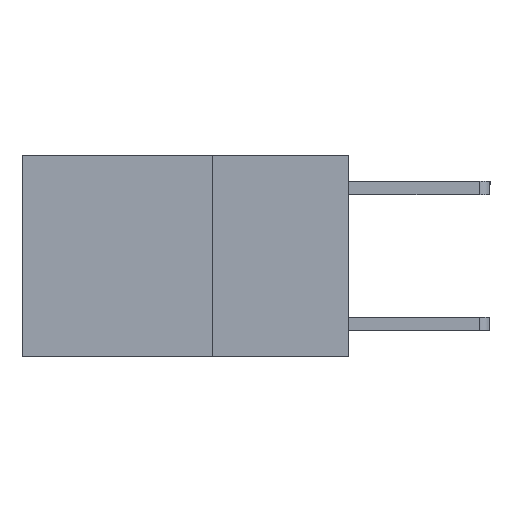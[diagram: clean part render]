
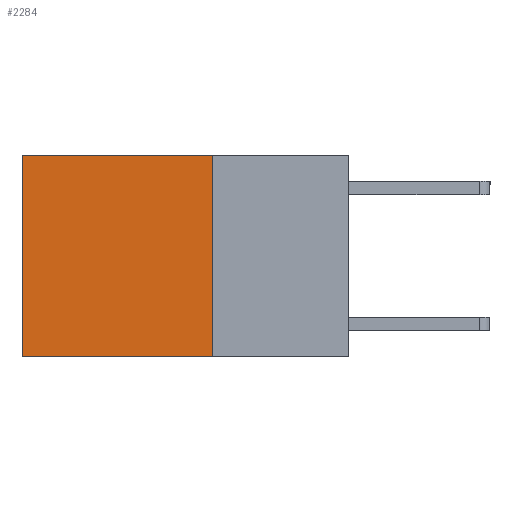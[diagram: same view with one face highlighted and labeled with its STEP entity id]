
A CAD part, left-side view. The second image highlights one B-rep face of the part: STEP entity #2284.
In plain terms, the highlighted planar face has unit normal (-1, 0, 0).
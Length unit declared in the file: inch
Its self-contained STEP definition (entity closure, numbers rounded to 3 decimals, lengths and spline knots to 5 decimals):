
#416 = EDGE_CURVE ( 'NONE', #8746, #8376, #2833, .T. ) ;
#611 = DIRECTION ( 'NONE',  ( 1., 0., 0. ) ) ;
#1203 = CARTESIAN_POINT ( 'NONE',  ( 0.2625, 0.25, 0. ) ) ;
#1419 = CARTESIAN_POINT ( 'NONE',  ( 0.2625, 0.25, -0.37 ) ) ;
#1579 = VECTOR ( 'NONE', #7755, 39.37008 ) ;
#1591 = ORIENTED_EDGE ( 'NONE', *, *, #10218, .F. ) ;
#2007 = LINE ( 'NONE', #1203, #3804 ) ;
#2231 = EDGE_LOOP ( 'NONE', ( #9813, #6695, #1591, #3372 ) ) ;
#2284 = ADVANCED_FACE ( 'NONE', ( #3762 ), #7117, .F. ) ;
#2610 = LINE ( 'NONE', #9349, #7134 ) ;
#2644 = CARTESIAN_POINT ( 'NONE',  ( 0.2625, 0.25, 0. ) ) ;
#2833 = LINE ( 'NONE', #7959, #8515 ) ;
#2939 = DIRECTION ( 'NONE',  ( 0., 1., 0. ) ) ;
#2969 = DIRECTION ( 'NONE',  ( 0., 0., -1. ) ) ;
#3318 = VERTEX_POINT ( 'NONE', #6523 ) ;
#3368 = DIRECTION ( 'NONE',  ( 0., 0., -1. ) ) ;
#3372 = ORIENTED_EDGE ( 'NONE', *, *, #6513, .T. ) ;
#3762 = FACE_OUTER_BOUND ( 'NONE', #2231, .T. ) ;
#3804 = VECTOR ( 'NONE', #5330, 39.37008 ) ;
#4680 = EDGE_CURVE ( 'NONE', #3318, #8376, #2610, .T. ) ;
#4691 = CARTESIAN_POINT ( 'NONE',  ( 0.2625, 0.25, 0. ) ) ;
#5330 = DIRECTION ( 'NONE',  ( 0., 1., 0. ) ) ;
#5818 = CARTESIAN_POINT ( 'NONE',  ( 0.2625, 0.25, 0. ) ) ;
#5992 = LINE ( 'NONE', #5818, #1579 ) ;
#6513 = EDGE_CURVE ( 'NONE', #8115, #3318, #2007, .T. ) ;
#6523 = CARTESIAN_POINT ( 'NONE',  ( 0.2625, 0.6, 0. ) ) ;
#6695 = ORIENTED_EDGE ( 'NONE', *, *, #416, .F. ) ;
#7117 = PLANE ( 'NONE',  #10668 ) ;
#7134 = VECTOR ( 'NONE', #3368, 39.37008 ) ;
#7755 = DIRECTION ( 'NONE',  ( 0., 0., -1. ) ) ;
#7959 = CARTESIAN_POINT ( 'NONE',  ( 0.2625, 0.25, -0.37 ) ) ;
#8115 = VERTEX_POINT ( 'NONE', #2644 ) ;
#8376 = VERTEX_POINT ( 'NONE', #9030 ) ;
#8515 = VECTOR ( 'NONE', #2939, 39.37008 ) ;
#8746 = VERTEX_POINT ( 'NONE', #1419 ) ;
#9030 = CARTESIAN_POINT ( 'NONE',  ( 0.2625, 0.6, -0.37 ) ) ;
#9349 = CARTESIAN_POINT ( 'NONE',  ( 0.2625, 0.6, 0. ) ) ;
#9813 = ORIENTED_EDGE ( 'NONE', *, *, #4680, .T. ) ;
#10218 = EDGE_CURVE ( 'NONE', #8115, #8746, #5992, .T. ) ;
#10668 = AXIS2_PLACEMENT_3D ( 'NONE', #4691, #611, #2969 ) ;
